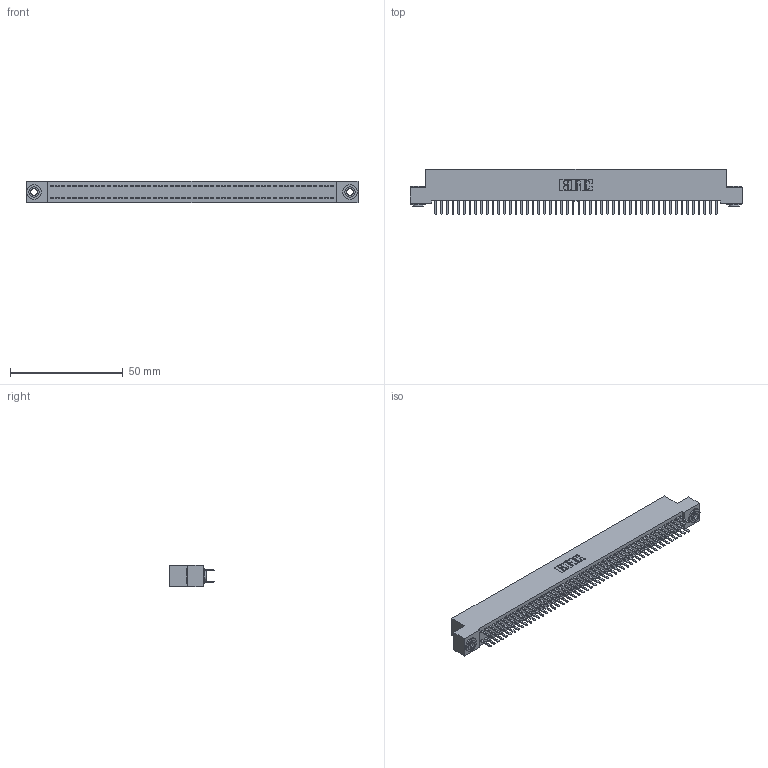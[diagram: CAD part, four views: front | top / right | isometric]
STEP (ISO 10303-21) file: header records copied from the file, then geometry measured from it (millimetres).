
FILE_DESCRIPTION (( 'STEP AP203' ), '1' );
FILE_NAME ('392-100-520-203.STEP', '2019-10-09T20:41:12', ( '' ), ( '' ), 'SwSTEP 2.0', 'SolidWorks 2016', '' );
FILE_SCHEMA (( 'CONFIG_CONTROL_DESIGN' ));
Length unit declared in the file: inch
Products named in the file (4): 345-292-001_345-293-120; 342-250-002_345-250-002-102; 392-100-520-203; 342 Part_.156 TH
Assembly tree (103 placements, depth 2):
  392-100-520-203
    342 Part_.156 TH
    345-292-001_345-293-120  x100
    342-250-002_345-250-002-102  x2
Bounding box: 147.32 x 20.02 x 9.4 mm (x, y, z)
Volume: 13253.4 mm3; surface area: 21880.7 mm2
Topology: 103 solids, 103 shells, 5748 faces, 16675 edges, 10846 vertices
Faces by surface type: plane 3876, cylinder 1864, cone 8
Entity records: 31764 total; most frequent: CARTESIAN_POINT 5241, ORIENTED_EDGE 5158, DIRECTION 4485, EDGE_CURVE 2579, LINE 2423, VECTOR 2423, VERTEX_POINT 1714, AXIS2_PLACEMENT_3D 1031
